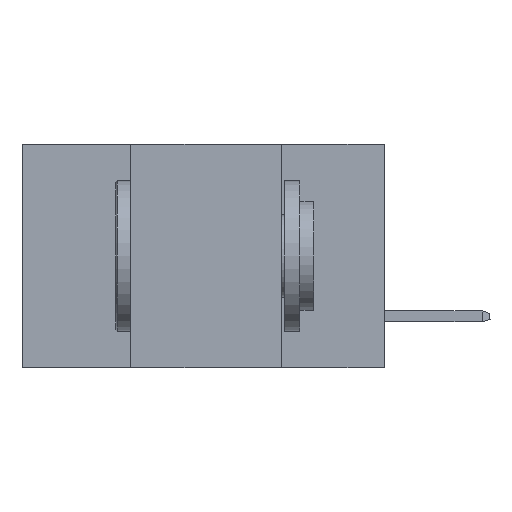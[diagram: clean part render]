
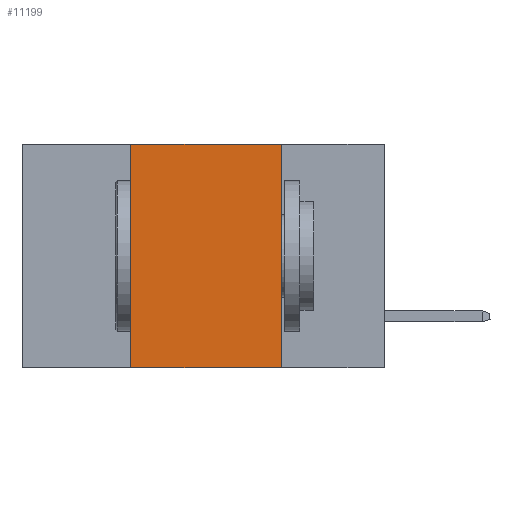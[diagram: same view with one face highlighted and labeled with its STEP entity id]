
A CAD part, left-side view. The second image highlights one B-rep face of the part: STEP entity #11199.
In plain terms, the highlighted planar face has unit normal (-1, 0, 0).
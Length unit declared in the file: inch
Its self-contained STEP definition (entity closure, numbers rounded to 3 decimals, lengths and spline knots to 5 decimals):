
#302 = ORIENTED_EDGE ( 'NONE', *, *, #27986, .T. ) ;
#365 = VECTOR ( 'NONE', #15553, 39.37008 ) ;
#1349 = VECTOR ( 'NONE', #24045, 39.37008 ) ;
#2371 = VECTOR ( 'NONE', #18387, 39.37008 ) ;
#2621 = EDGE_CURVE ( 'NONE', #9333, #21607, #12447, .T. ) ;
#4349 = VERTEX_POINT ( 'NONE', #17603 ) ;
#4455 = LINE ( 'NONE', #25958, #2371 ) ;
#4484 = DIRECTION ( 'NONE',  ( 0., 0., -1. ) ) ;
#5868 = LINE ( 'NONE', #26226, #12380 ) ;
#6188 = EDGE_CURVE ( 'NONE', #21607, #10348, #4455, .T. ) ;
#6296 = CARTESIAN_POINT ( 'NONE',  ( 0., 0.17, -0.37 ) ) ;
#9333 = VERTEX_POINT ( 'NONE', #13901 ) ;
#10348 = VERTEX_POINT ( 'NONE', #6296 ) ;
#10639 = EDGE_LOOP ( 'NONE', ( #12241, #26668, #20374, #302 ) ) ;
#11199 = ADVANCED_FACE ( 'NONE', ( #11350 ), #17541, .F. ) ;
#11350 = FACE_OUTER_BOUND ( 'NONE', #10639, .T. ) ;
#12241 = ORIENTED_EDGE ( 'NONE', *, *, #6188, .F. ) ;
#12380 = VECTOR ( 'NONE', #19730, 39.37008 ) ;
#12447 = LINE ( 'NONE', #17484, #365 ) ;
#13901 = CARTESIAN_POINT ( 'NONE',  ( 0., 0.42, 0. ) ) ;
#15243 = DIRECTION ( 'NONE',  ( 1., 0., 0. ) ) ;
#15553 = DIRECTION ( 'NONE',  ( 0., -1., 0. ) ) ;
#15573 = EDGE_CURVE ( 'NONE', #4349, #9333, #5868, .T. ) ;
#17184 = LINE ( 'NONE', #26157, #1349 ) ;
#17484 = CARTESIAN_POINT ( 'NONE',  ( 0., 0.6, 0. ) ) ;
#17541 = PLANE ( 'NONE',  #20786 ) ;
#17603 = CARTESIAN_POINT ( 'NONE',  ( 0., 0.42, -0.37 ) ) ;
#18387 = DIRECTION ( 'NONE',  ( 0., 0., -1. ) ) ;
#18885 = CARTESIAN_POINT ( 'NONE',  ( 0., 0.17, 0. ) ) ;
#19629 = CARTESIAN_POINT ( 'NONE',  ( 0., 0.6, 0. ) ) ;
#19730 = DIRECTION ( 'NONE',  ( 0., 0., 1. ) ) ;
#20374 = ORIENTED_EDGE ( 'NONE', *, *, #15573, .F. ) ;
#20786 = AXIS2_PLACEMENT_3D ( 'NONE', #19629, #15243, #4484 ) ;
#21607 = VERTEX_POINT ( 'NONE', #18885 ) ;
#24045 = DIRECTION ( 'NONE',  ( 0., -1., 0. ) ) ;
#25958 = CARTESIAN_POINT ( 'NONE',  ( 0., 0.17, 0. ) ) ;
#26157 = CARTESIAN_POINT ( 'NONE',  ( 0., 0.6, -0.37 ) ) ;
#26226 = CARTESIAN_POINT ( 'NONE',  ( 0., 0.42, 0. ) ) ;
#26668 = ORIENTED_EDGE ( 'NONE', *, *, #2621, .F. ) ;
#27986 = EDGE_CURVE ( 'NONE', #4349, #10348, #17184, .T. ) ;
